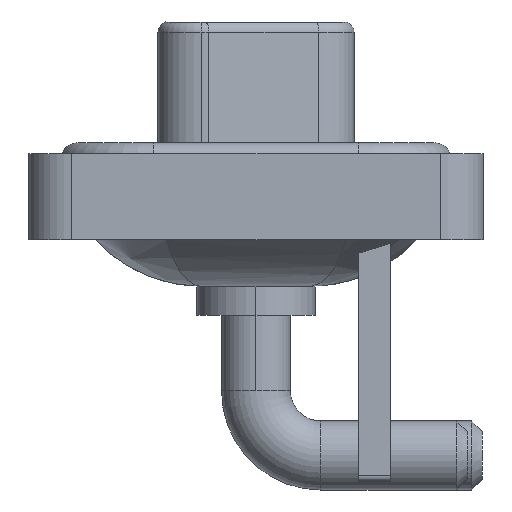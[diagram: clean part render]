
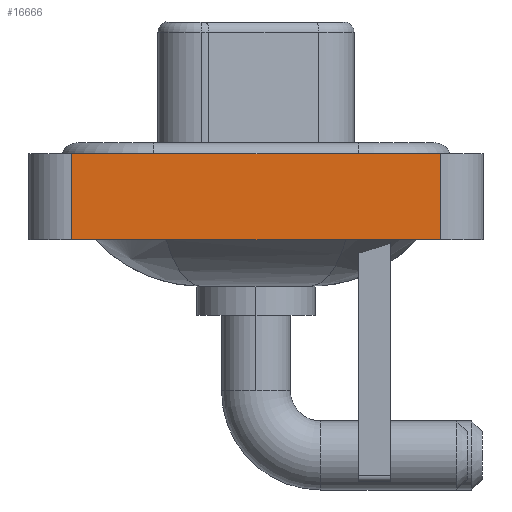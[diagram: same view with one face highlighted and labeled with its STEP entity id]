
A CAD part, left-side view. The second image highlights one B-rep face of the part: STEP entity #16666.
In plain terms, the highlighted planar face has unit normal (-1, 0, 0).
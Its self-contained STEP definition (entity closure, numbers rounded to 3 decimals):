
#30 = VECTOR ( 'NONE', #10186, 1000. ) ;
#521 = CARTESIAN_POINT ( 'NONE',  ( -7.3, -8.55, 0.4 ) ) ;
#564 = FACE_OUTER_BOUND ( 'NONE', #6258, .T. ) ;
#1647 = DIRECTION ( 'NONE',  ( 0., -1., 0. ) ) ;
#1960 = EDGE_CURVE ( 'NONE', #3672, #7798, #15517, .T. ) ;
#2061 = EDGE_CURVE ( 'NONE', #9445, #4315, #3809, .T. ) ;
#2379 = ORIENTED_EDGE ( 'NONE', *, *, #1960, .F. ) ;
#3672 = VERTEX_POINT ( 'NONE', #6256 ) ;
#3719 = CARTESIAN_POINT ( 'NONE',  ( -7.3, -8.55, -3.6 ) ) ;
#3809 = LINE ( 'NONE', #3719, #30 ) ;
#4315 = VERTEX_POINT ( 'NONE', #521 ) ;
#4364 = DIRECTION ( 'NONE',  ( 0., 0., 1. ) ) ;
#4692 = CARTESIAN_POINT ( 'NONE',  ( -7.3, -8.55, 0.4 ) ) ;
#6202 = DIRECTION ( 'NONE',  ( 0., -1., 0. ) ) ;
#6256 = CARTESIAN_POINT ( 'NONE',  ( -7.3, 8.55, -3.6 ) ) ;
#6258 = EDGE_LOOP ( 'NONE', ( #7073, #12160, #2379, #10017 ) ) ;
#6301 = LINE ( 'NONE', #4692, #11158 ) ;
#6509 = CARTESIAN_POINT ( 'NONE',  ( -7.3, -8.55, -3.6 ) ) ;
#7073 = ORIENTED_EDGE ( 'NONE', *, *, #2061, .T. ) ;
#7798 = VERTEX_POINT ( 'NONE', #12401 ) ;
#8026 = LINE ( 'NONE', #6509, #16754 ) ;
#9445 = VERTEX_POINT ( 'NONE', #14551 ) ;
#10017 = ORIENTED_EDGE ( 'NONE', *, *, #15895, .T. ) ;
#10186 = DIRECTION ( 'NONE',  ( 0., 0., 1. ) ) ;
#10271 = AXIS2_PLACEMENT_3D ( 'NONE', #13036, #12832, #19231 ) ;
#11158 = VECTOR ( 'NONE', #6202, 1000. ) ;
#12160 = ORIENTED_EDGE ( 'NONE', *, *, #14654, .F. ) ;
#12306 = VECTOR ( 'NONE', #4364, 1000. ) ;
#12401 = CARTESIAN_POINT ( 'NONE',  ( -7.3, 8.55, 0.4 ) ) ;
#12832 = DIRECTION ( 'NONE',  ( -1., 0., 0. ) ) ;
#13036 = CARTESIAN_POINT ( 'NONE',  ( -7.3, -8.55, -3.6 ) ) ;
#14357 = PLANE ( 'NONE',  #10271 ) ;
#14551 = CARTESIAN_POINT ( 'NONE',  ( -7.3, -8.55, -3.6 ) ) ;
#14654 = EDGE_CURVE ( 'NONE', #7798, #4315, #6301, .T. ) ;
#15517 = LINE ( 'NONE', #16957, #12306 ) ;
#15895 = EDGE_CURVE ( 'NONE', #3672, #9445, #8026, .T. ) ;
#16666 = ADVANCED_FACE ( 'NONE', ( #564 ), #14357, .T. ) ;
#16754 = VECTOR ( 'NONE', #1647, 1000. ) ;
#16957 = CARTESIAN_POINT ( 'NONE',  ( -7.3, 8.55, -3.6 ) ) ;
#19231 = DIRECTION ( 'NONE',  ( 0., 0., 1. ) ) ;
